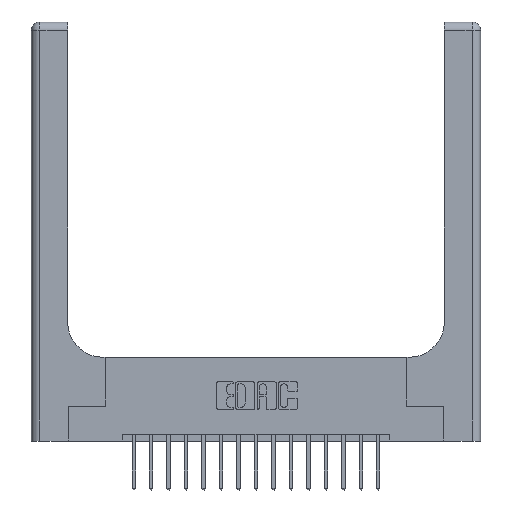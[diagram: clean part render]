
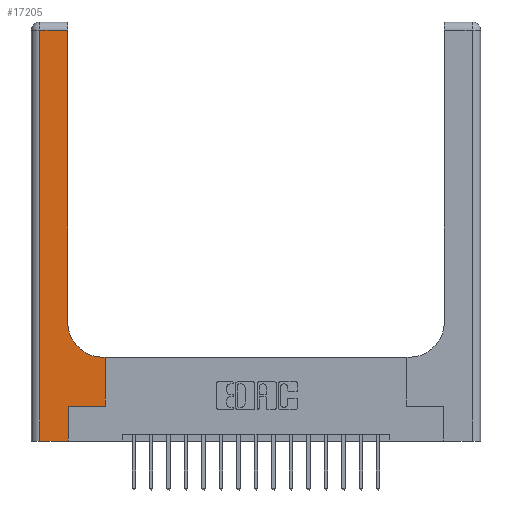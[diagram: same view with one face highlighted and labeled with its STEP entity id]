
A CAD part, top view. The second image highlights one B-rep face of the part: STEP entity #17205.
In plain terms, the highlighted planar face has unit normal (0, 0, 1).
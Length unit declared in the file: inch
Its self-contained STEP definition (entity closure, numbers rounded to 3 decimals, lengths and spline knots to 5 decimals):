
#128 = AXIS2_PLACEMENT_3D ( 'NONE', #12203, #3236, #12007 ) ;
#394 = CARTESIAN_POINT ( 'NONE',  ( 0.528, 0.25, 0.37 ) ) ;
#447 = LINE ( 'NONE', #3056, #12661 ) ;
#834 = EDGE_CURVE ( 'NONE', #17584, #8279, #7431, .T. ) ;
#929 = VECTOR ( 'NONE', #12932, 39.37008 ) ;
#1368 = ORIENTED_EDGE ( 'NONE', *, *, #9019, .T. ) ;
#1369 = VECTOR ( 'NONE', #4892, 39.37008 ) ;
#1447 = LINE ( 'NONE', #7963, #1369 ) ;
#1935 = EDGE_CURVE ( 'NONE', #6589, #18416, #12501, .T. ) ;
#2110 = ORIENTED_EDGE ( 'NONE', *, *, #1935, .T. ) ;
#2441 = ORIENTED_EDGE ( 'NONE', *, *, #2522, .T. ) ;
#2522 = EDGE_CURVE ( 'NONE', #17312, #8197, #2913, .T. ) ;
#2906 = LINE ( 'NONE', #4532, #16101 ) ;
#2913 = LINE ( 'NONE', #3011, #929 ) ;
#3011 = CARTESIAN_POINT ( 'NONE',  ( 0.265, 0.25, 0.37 ) ) ;
#3056 = CARTESIAN_POINT ( 'NONE',  ( 0.265, 0., 0.37 ) ) ;
#3236 = DIRECTION ( 'NONE',  ( 0., 0., -1. ) ) ;
#4505 = CARTESIAN_POINT ( 'NONE',  ( 0.528, 0.6, 0.37 ) ) ;
#4532 = CARTESIAN_POINT ( 'NONE',  ( 0.528, 0.25, 0.37 ) ) ;
#4655 = EDGE_CURVE ( 'NONE', #11559, #17312, #447, .T. ) ;
#4769 = CARTESIAN_POINT ( 'NONE',  ( 0.26, 3., 0.37 ) ) ;
#4892 = DIRECTION ( 'NONE',  ( 1., 0., 0. ) ) ;
#5029 = CARTESIAN_POINT ( 'NONE',  ( 0.265, 0.25, 0.37 ) ) ;
#5032 = CARTESIAN_POINT ( 'NONE',  ( 0.06, 0., 0.37 ) ) ;
#5114 = ORIENTED_EDGE ( 'NONE', *, *, #4655, .T. ) ;
#5255 = VECTOR ( 'NONE', #17785, 39.37008 ) ;
#6027 = CARTESIAN_POINT ( 'NONE',  ( 0.51, 0.6, 0.37 ) ) ;
#6419 = DIRECTION ( 'NONE',  ( -1., 0., 0. ) ) ;
#6470 = DIRECTION ( 'NONE',  ( -1., 0., 0. ) ) ;
#6589 = VERTEX_POINT ( 'NONE', #4505 ) ;
#7025 = VECTOR ( 'NONE', #6419, 39.37008 ) ;
#7321 = DIRECTION ( 'NONE',  ( 0., 1., 0. ) ) ;
#7431 = LINE ( 'NONE', #11875, #5255 ) ;
#7765 = ORIENTED_EDGE ( 'NONE', *, *, #10310, .T. ) ;
#7963 = CARTESIAN_POINT ( 'NONE',  ( 0., 0., 0.37 ) ) ;
#8111 = DIRECTION ( 'NONE',  ( 0., 0., -1. ) ) ;
#8197 = VERTEX_POINT ( 'NONE', #394 ) ;
#8279 = VERTEX_POINT ( 'NONE', #16791 ) ;
#8701 = ORIENTED_EDGE ( 'NONE', *, *, #834, .T. ) ;
#9019 = EDGE_CURVE ( 'NONE', #8279, #9055, #17020, .T. ) ;
#9055 = VERTEX_POINT ( 'NONE', #5032 ) ;
#9822 = EDGE_CURVE ( 'NONE', #9055, #11559, #1447, .T. ) ;
#10310 = EDGE_CURVE ( 'NONE', #18416, #17161, #12453, .T. ) ;
#10715 = FACE_OUTER_BOUND ( 'NONE', #15858, .T. ) ;
#10942 = ORIENTED_EDGE ( 'NONE', *, *, #17485, .T. ) ;
#11009 = DIRECTION ( 'NONE',  ( 0., -1., 0. ) ) ;
#11102 = PLANE ( 'NONE',  #13321 ) ;
#11559 = VERTEX_POINT ( 'NONE', #17560 ) ;
#11875 = CARTESIAN_POINT ( 'NONE',  ( 0., 2.94, 0.37 ) ) ;
#11957 = CARTESIAN_POINT ( 'NONE',  ( 0.26, 2.94, 0.37 ) ) ;
#12007 = DIRECTION ( 'NONE',  ( 1., 0., 0. ) ) ;
#12203 = CARTESIAN_POINT ( 'NONE',  ( 0.51, 0.85, 0.37 ) ) ;
#12453 = CIRCLE ( 'NONE', #128, 0.25 ) ;
#12501 = LINE ( 'NONE', #17060, #7025 ) ;
#12639 = ORIENTED_EDGE ( 'NONE', *, *, #16652, .T. ) ;
#12661 = VECTOR ( 'NONE', #15004, 39.37008 ) ;
#12932 = DIRECTION ( 'NONE',  ( 1., 0., 0. ) ) ;
#13321 = AXIS2_PLACEMENT_3D ( 'NONE', #13708, #8111, #6470 ) ;
#13708 = CARTESIAN_POINT ( 'NONE',  ( 0., 3., 0.37 ) ) ;
#14141 = ORIENTED_EDGE ( 'NONE', *, *, #9822, .T. ) ;
#14610 = LINE ( 'NONE', #4769, #18260 ) ;
#15004 = DIRECTION ( 'NONE',  ( 0., 1., 0. ) ) ;
#15350 = CARTESIAN_POINT ( 'NONE',  ( 0.06, 3., 0.37 ) ) ;
#15858 = EDGE_LOOP ( 'NONE', ( #12639, #8701, #1368, #14141, #5114, #2441, #10942, #2110, #7765 ) ) ;
#16101 = VECTOR ( 'NONE', #7321, 39.37008 ) ;
#16160 = VECTOR ( 'NONE', #11009, 39.37008 ) ;
#16259 = DIRECTION ( 'NONE',  ( 0., 1., 0. ) ) ;
#16422 = CARTESIAN_POINT ( 'NONE',  ( 0.26, 0.85, 0.37 ) ) ;
#16652 = EDGE_CURVE ( 'NONE', #17161, #17584, #14610, .T. ) ;
#16791 = CARTESIAN_POINT ( 'NONE',  ( 0.06, 2.94, 0.37 ) ) ;
#17020 = LINE ( 'NONE', #15350, #16160 ) ;
#17060 = CARTESIAN_POINT ( 'NONE',  ( 0.26, 0.6, 0.37 ) ) ;
#17161 = VERTEX_POINT ( 'NONE', #16422 ) ;
#17205 = ADVANCED_FACE ( 'NONE', ( #10715 ), #11102, .F. ) ;
#17312 = VERTEX_POINT ( 'NONE', #5029 ) ;
#17485 = EDGE_CURVE ( 'NONE', #8197, #6589, #2906, .T. ) ;
#17560 = CARTESIAN_POINT ( 'NONE',  ( 0.265, 0., 0.37 ) ) ;
#17584 = VERTEX_POINT ( 'NONE', #11957 ) ;
#17785 = DIRECTION ( 'NONE',  ( -1., 0., 0. ) ) ;
#18260 = VECTOR ( 'NONE', #16259, 39.37008 ) ;
#18416 = VERTEX_POINT ( 'NONE', #6027 ) ;
